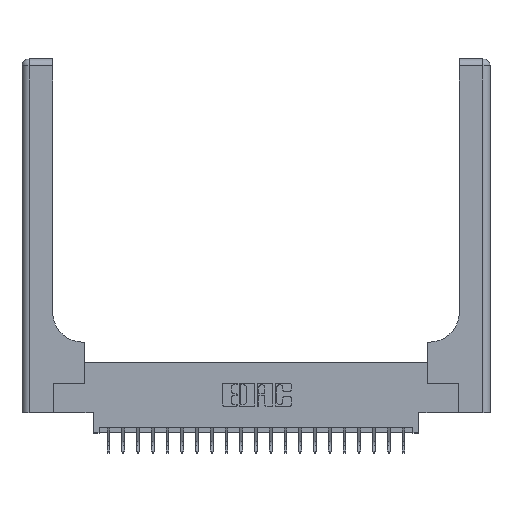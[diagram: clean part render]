
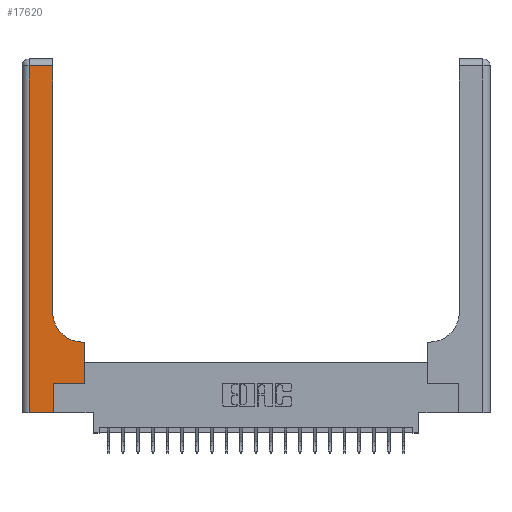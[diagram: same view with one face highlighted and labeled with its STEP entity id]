
A CAD part, top view. The second image highlights one B-rep face of the part: STEP entity #17620.
In plain terms, the highlighted planar face has unit normal (0, 0, 1).
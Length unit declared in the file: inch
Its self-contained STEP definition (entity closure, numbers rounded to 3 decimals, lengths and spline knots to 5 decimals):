
#188 = VERTEX_POINT ( 'NONE', #3162 ) ;
#207 = DIRECTION ( 'NONE',  ( 0., -1., 0. ) ) ;
#313 = VECTOR ( 'NONE', #7386, 39.37008 ) ;
#480 = VECTOR ( 'NONE', #16045, 39.37008 ) ;
#751 = LINE ( 'NONE', #21500, #21042 ) ;
#1288 = CARTESIAN_POINT ( 'NONE',  ( 0.528, 0.6, 0.37 ) ) ;
#1352 = LINE ( 'NONE', #20157, #21282 ) ;
#1550 = ORIENTED_EDGE ( 'NONE', *, *, #22321, .T. ) ;
#1809 = CARTESIAN_POINT ( 'NONE',  ( 0.265, 0.25, 0.37 ) ) ;
#1896 = ORIENTED_EDGE ( 'NONE', *, *, #5599, .T. ) ;
#2180 = ORIENTED_EDGE ( 'NONE', *, *, #18010, .T. ) ;
#2300 = VERTEX_POINT ( 'NONE', #17874 ) ;
#2354 = CARTESIAN_POINT ( 'NONE',  ( 0.265, 0.25, 0.37 ) ) ;
#2398 = ORIENTED_EDGE ( 'NONE', *, *, #2550, .T. ) ;
#2550 = EDGE_CURVE ( 'NONE', #17894, #188, #19690, .T. ) ;
#2574 = ORIENTED_EDGE ( 'NONE', *, *, #12881, .T. ) ;
#2598 = AXIS2_PLACEMENT_3D ( 'NONE', #15871, #7214, #7331 ) ;
#2985 = VERTEX_POINT ( 'NONE', #1288 ) ;
#3162 = CARTESIAN_POINT ( 'NONE',  ( 0.528, 0.25, 0.37 ) ) ;
#3436 = ORIENTED_EDGE ( 'NONE', *, *, #19805, .T. ) ;
#3739 = VERTEX_POINT ( 'NONE', #4965 ) ;
#3851 = EDGE_CURVE ( 'NONE', #11818, #18017, #4853, .T. ) ;
#4071 = CIRCLE ( 'NONE', #2598, 0.25 ) ;
#4756 = CARTESIAN_POINT ( 'NONE',  ( 0.06, 0., 0.37 ) ) ;
#4853 = LINE ( 'NONE', #15220, #11587 ) ;
#4965 = CARTESIAN_POINT ( 'NONE',  ( 0.06, 2.94, 0.37 ) ) ;
#5599 = EDGE_CURVE ( 'NONE', #15854, #11818, #4071, .T. ) ;
#5670 = LINE ( 'NONE', #10592, #313 ) ;
#6031 = DIRECTION ( 'NONE',  ( 0., 1., 0. ) ) ;
#6577 = VECTOR ( 'NONE', #9312, 39.37008 ) ;
#7214 = DIRECTION ( 'NONE',  ( 0., 0., -1. ) ) ;
#7331 = DIRECTION ( 'NONE',  ( 1., 0., 0. ) ) ;
#7386 = DIRECTION ( 'NONE',  ( -1., 0., 0. ) ) ;
#7494 = LINE ( 'NONE', #9318, #480 ) ;
#7595 = EDGE_CURVE ( 'NONE', #18017, #3739, #7494, .T. ) ;
#8510 = DIRECTION ( 'NONE',  ( 0., 1., 0. ) ) ;
#9106 = EDGE_CURVE ( 'NONE', #188, #2985, #1352, .T. ) ;
#9312 = DIRECTION ( 'NONE',  ( 1., 0., 0. ) ) ;
#9318 = CARTESIAN_POINT ( 'NONE',  ( 0., 2.94, 0.37 ) ) ;
#10592 = CARTESIAN_POINT ( 'NONE',  ( 0.26, 0.6, 0.37 ) ) ;
#11587 = VECTOR ( 'NONE', #8510, 39.37008 ) ;
#11818 = VERTEX_POINT ( 'NONE', #12849 ) ;
#12849 = CARTESIAN_POINT ( 'NONE',  ( 0.26, 0.85, 0.37 ) ) ;
#12881 = EDGE_CURVE ( 'NONE', #3739, #13261, #17210, .T. ) ;
#12991 = VECTOR ( 'NONE', #207, 39.37008 ) ;
#13261 = VERTEX_POINT ( 'NONE', #4756 ) ;
#14139 = DIRECTION ( 'NONE',  ( 0., 0., -1. ) ) ;
#15220 = CARTESIAN_POINT ( 'NONE',  ( 0.26, 3., 0.37 ) ) ;
#15836 = CARTESIAN_POINT ( 'NONE',  ( 0., 3., 0.37 ) ) ;
#15854 = VERTEX_POINT ( 'NONE', #19633 ) ;
#15871 = CARTESIAN_POINT ( 'NONE',  ( 0.51, 0.85, 0.37 ) ) ;
#16045 = DIRECTION ( 'NONE',  ( -1., 0., 0. ) ) ;
#16296 = FACE_OUTER_BOUND ( 'NONE', #22197, .T. ) ;
#17086 = DIRECTION ( 'NONE',  ( 0., 1., 0. ) ) ;
#17210 = LINE ( 'NONE', #22434, #12991 ) ;
#17325 = ORIENTED_EDGE ( 'NONE', *, *, #9106, .T. ) ;
#17540 = CARTESIAN_POINT ( 'NONE',  ( 0.26, 2.94, 0.37 ) ) ;
#17620 = ADVANCED_FACE ( 'NONE', ( #16296 ), #19380, .F. ) ;
#17874 = CARTESIAN_POINT ( 'NONE',  ( 0.265, 0., 0.37 ) ) ;
#17894 = VERTEX_POINT ( 'NONE', #1809 ) ;
#18010 = EDGE_CURVE ( 'NONE', #2985, #15854, #5670, .T. ) ;
#18017 = VERTEX_POINT ( 'NONE', #17540 ) ;
#18052 = VECTOR ( 'NONE', #6031, 39.37008 ) ;
#19223 = ORIENTED_EDGE ( 'NONE', *, *, #3851, .T. ) ;
#19380 = PLANE ( 'NONE',  #20757 ) ;
#19633 = CARTESIAN_POINT ( 'NONE',  ( 0.51, 0.6, 0.37 ) ) ;
#19678 = DIRECTION ( 'NONE',  ( 1., 0., 0. ) ) ;
#19690 = LINE ( 'NONE', #2354, #6577 ) ;
#19805 = EDGE_CURVE ( 'NONE', #2300, #17894, #21644, .T. ) ;
#20157 = CARTESIAN_POINT ( 'NONE',  ( 0.528, 0.25, 0.37 ) ) ;
#20204 = ORIENTED_EDGE ( 'NONE', *, *, #7595, .T. ) ;
#20757 = AXIS2_PLACEMENT_3D ( 'NONE', #15836, #14139, #21200 ) ;
#21042 = VECTOR ( 'NONE', #19678, 39.37008 ) ;
#21200 = DIRECTION ( 'NONE',  ( -1., 0., 0. ) ) ;
#21282 = VECTOR ( 'NONE', #17086, 39.37008 ) ;
#21420 = CARTESIAN_POINT ( 'NONE',  ( 0.265, 0., 0.37 ) ) ;
#21500 = CARTESIAN_POINT ( 'NONE',  ( 0., 0., 0.37 ) ) ;
#21644 = LINE ( 'NONE', #21420, #18052 ) ;
#22197 = EDGE_LOOP ( 'NONE', ( #19223, #20204, #2574, #1550, #3436, #2398, #17325, #2180, #1896 ) ) ;
#22321 = EDGE_CURVE ( 'NONE', #13261, #2300, #751, .T. ) ;
#22434 = CARTESIAN_POINT ( 'NONE',  ( 0.06, 3., 0.37 ) ) ;
